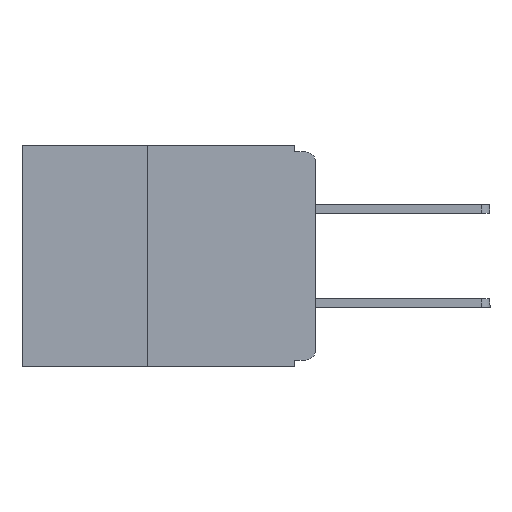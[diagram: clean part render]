
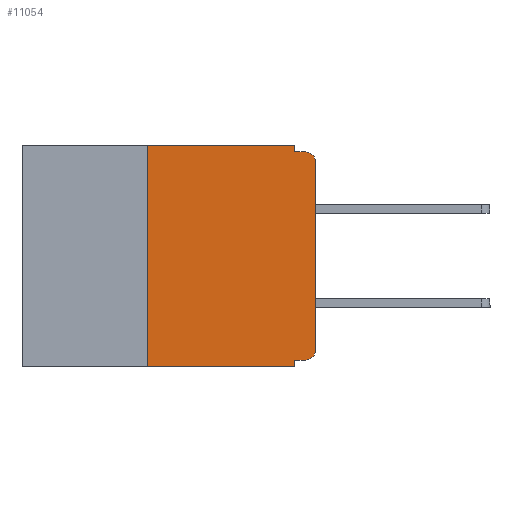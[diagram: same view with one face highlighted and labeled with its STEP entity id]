
A CAD part, left-side view. The second image highlights one B-rep face of the part: STEP entity #11054.
In plain terms, the highlighted planar face has unit normal (-1, 0, 0).
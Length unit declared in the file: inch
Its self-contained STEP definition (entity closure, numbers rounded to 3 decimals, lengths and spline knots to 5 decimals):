
#98 = AXIS2_PLACEMENT_3D ( 'NONE', #13664, #13645, #13628 ) ;
#144 = VERTEX_POINT ( 'NONE', #2262 ) ;
#265 = ORIENTED_EDGE ( 'NONE', *, *, #3256, .F. ) ;
#276 = CIRCLE ( 'NONE', #98, 0.015 ) ;
#456 = ORIENTED_EDGE ( 'NONE', *, *, #9646, .F. ) ;
#1357 = VERTEX_POINT ( 'NONE', #14803 ) ;
#1540 = EDGE_CURVE ( 'NONE', #7897, #1597, #4704, .T. ) ;
#1597 = VERTEX_POINT ( 'NONE', #12287 ) ;
#2142 = CARTESIAN_POINT ( 'NONE',  ( 0., 0.437, 0. ) ) ;
#2262 = CARTESIAN_POINT ( 'NONE',  ( 0., 0.25, -0.33 ) ) ;
#2383 = CARTESIAN_POINT ( 'NONE',  ( 0., 0.031, -0.33 ) ) ;
#2394 = ORIENTED_EDGE ( 'NONE', *, *, #3773, .F. ) ;
#2497 = VECTOR ( 'NONE', #9174, 39.37008 ) ;
#2506 = PLANE ( 'NONE',  #11455 ) ;
#2743 = DIRECTION ( 'NONE',  ( 0., -1., 0. ) ) ;
#3132 = DIRECTION ( 'NONE',  ( 0., -1., 0. ) ) ;
#3256 = EDGE_CURVE ( 'NONE', #144, #6003, #4223, .T. ) ;
#3603 = CARTESIAN_POINT ( 'NONE',  ( 0., 0.437, -0.33 ) ) ;
#3773 = EDGE_CURVE ( 'NONE', #6003, #5235, #4430, .T. ) ;
#3990 = LINE ( 'NONE', #15633, #6491 ) ;
#4163 = VECTOR ( 'NONE', #12438, 39.37008 ) ;
#4223 = LINE ( 'NONE', #7799, #10571 ) ;
#4293 = CARTESIAN_POINT ( 'NONE',  ( 0., 0.031, -0.32 ) ) ;
#4430 = LINE ( 'NONE', #2142, #10390 ) ;
#4597 = VERTEX_POINT ( 'NONE', #10566 ) ;
#4655 = DIRECTION ( 'NONE',  ( 0., 0., 1. ) ) ;
#4704 = LINE ( 'NONE', #7471, #13561 ) ;
#4979 = LINE ( 'NONE', #6855, #7892 ) ;
#5074 = EDGE_CURVE ( 'NONE', #13038, #7530, #3990, .T. ) ;
#5094 = DIRECTION ( 'NONE',  ( 1., 0., 0. ) ) ;
#5200 = DIRECTION ( 'NONE',  ( -1., 0., 0. ) ) ;
#5235 = VERTEX_POINT ( 'NONE', #14043 ) ;
#5275 = EDGE_CURVE ( 'NONE', #14091, #7897, #276, .T. ) ;
#5726 = EDGE_CURVE ( 'NONE', #14091, #13038, #9710, .T. ) ;
#5735 = DIRECTION ( 'NONE',  ( 0., 0., 1. ) ) ;
#6003 = VERTEX_POINT ( 'NONE', #6795 ) ;
#6170 = ORIENTED_EDGE ( 'NONE', *, *, #11457, .T. ) ;
#6491 = VECTOR ( 'NONE', #15535, 39.37008 ) ;
#6626 = EDGE_LOOP ( 'NONE', ( #11677, #8546, #9915, #456, #2394, #265, #6170, #12557, #16315, #13457 ) ) ;
#6795 = CARTESIAN_POINT ( 'NONE',  ( 0., 0.25, 0. ) ) ;
#6855 = CARTESIAN_POINT ( 'NONE',  ( 0., 0., -0.01 ) ) ;
#7350 = CARTESIAN_POINT ( 'NONE',  ( 0., 0.031, 0. ) ) ;
#7445 = LINE ( 'NONE', #3603, #4163 ) ;
#7471 = CARTESIAN_POINT ( 'NONE',  ( 0., 0., 0. ) ) ;
#7530 = VERTEX_POINT ( 'NONE', #2383 ) ;
#7799 = CARTESIAN_POINT ( 'NONE',  ( 0., 0.25, -0.33 ) ) ;
#7892 = VECTOR ( 'NONE', #3132, 39.37008 ) ;
#7897 = VERTEX_POINT ( 'NONE', #15722 ) ;
#8148 = AXIS2_PLACEMENT_3D ( 'NONE', #12775, #5200, #14002 ) ;
#8546 = ORIENTED_EDGE ( 'NONE', *, *, #12882, .T. ) ;
#8927 = CARTESIAN_POINT ( 'NONE',  ( 0., 0.015, -0.32 ) ) ;
#9136 = CARTESIAN_POINT ( 'NONE',  ( 0., 0., -0.32 ) ) ;
#9174 = DIRECTION ( 'NONE',  ( 0., 1., 0. ) ) ;
#9475 = CIRCLE ( 'NONE', #8148, 0.015 ) ;
#9646 = EDGE_CURVE ( 'NONE', #5235, #4597, #10170, .T. ) ;
#9710 = LINE ( 'NONE', #9136, #2497 ) ;
#9915 = ORIENTED_EDGE ( 'NONE', *, *, #10048, .F. ) ;
#10048 = EDGE_CURVE ( 'NONE', #4597, #1357, #4979, .T. ) ;
#10170 = LINE ( 'NONE', #7350, #13085 ) ;
#10390 = VECTOR ( 'NONE', #2743, 39.37008 ) ;
#10566 = CARTESIAN_POINT ( 'NONE',  ( 0., 0.031, -0.01 ) ) ;
#10571 = VECTOR ( 'NONE', #4655, 39.37008 ) ;
#11054 = ADVANCED_FACE ( 'NONE', ( #13415 ), #2506, .F. ) ;
#11455 = AXIS2_PLACEMENT_3D ( 'NONE', #16280, #5094, #13902 ) ;
#11457 = EDGE_CURVE ( 'NONE', #144, #7530, #7445, .T. ) ;
#11677 = ORIENTED_EDGE ( 'NONE', *, *, #1540, .T. ) ;
#12287 = CARTESIAN_POINT ( 'NONE',  ( 0., 0., -0.025 ) ) ;
#12437 = DIRECTION ( 'NONE',  ( 0., 0., -1. ) ) ;
#12438 = DIRECTION ( 'NONE',  ( 0., -1., 0. ) ) ;
#12557 = ORIENTED_EDGE ( 'NONE', *, *, #5074, .F. ) ;
#12775 = CARTESIAN_POINT ( 'NONE',  ( 0., 0.015, -0.025 ) ) ;
#12882 = EDGE_CURVE ( 'NONE', #1597, #1357, #9475, .T. ) ;
#13038 = VERTEX_POINT ( 'NONE', #4293 ) ;
#13085 = VECTOR ( 'NONE', #12437, 39.37008 ) ;
#13415 = FACE_OUTER_BOUND ( 'NONE', #6626, .T. ) ;
#13457 = ORIENTED_EDGE ( 'NONE', *, *, #5275, .T. ) ;
#13561 = VECTOR ( 'NONE', #5735, 39.37008 ) ;
#13628 = DIRECTION ( 'NONE',  ( 0., 0., -1. ) ) ;
#13645 = DIRECTION ( 'NONE',  ( -1., 0., 0. ) ) ;
#13664 = CARTESIAN_POINT ( 'NONE',  ( 0., 0.015, -0.305 ) ) ;
#13902 = DIRECTION ( 'NONE',  ( 0., 0., -1. ) ) ;
#14002 = DIRECTION ( 'NONE',  ( 0., 0., -1. ) ) ;
#14043 = CARTESIAN_POINT ( 'NONE',  ( 0., 0.031, 0. ) ) ;
#14091 = VERTEX_POINT ( 'NONE', #8927 ) ;
#14803 = CARTESIAN_POINT ( 'NONE',  ( 0., 0.015, -0.01 ) ) ;
#15535 = DIRECTION ( 'NONE',  ( 0., 0., -1. ) ) ;
#15633 = CARTESIAN_POINT ( 'NONE',  ( 0., 0.031, -0.33 ) ) ;
#15722 = CARTESIAN_POINT ( 'NONE',  ( 0., 0., -0.305 ) ) ;
#16280 = CARTESIAN_POINT ( 'NONE',  ( 0., 0.437, 0. ) ) ;
#16315 = ORIENTED_EDGE ( 'NONE', *, *, #5726, .F. ) ;
